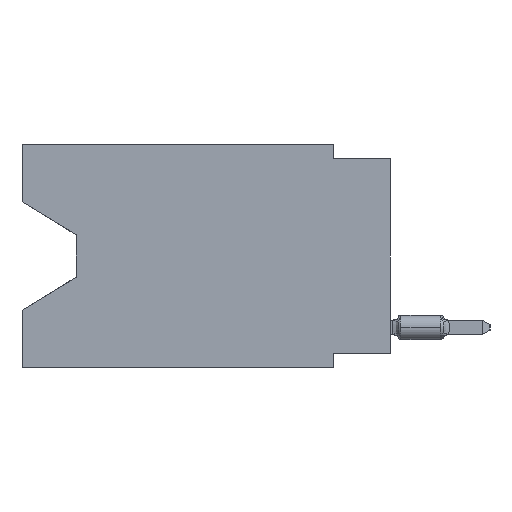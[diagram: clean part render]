
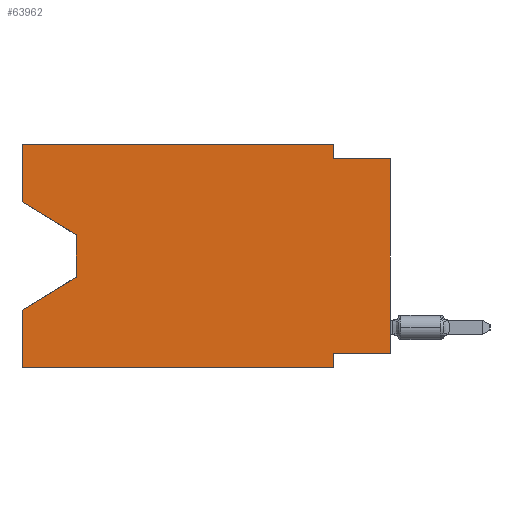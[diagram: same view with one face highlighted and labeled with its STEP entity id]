
A CAD part, left-side view. The second image highlights one B-rep face of the part: STEP entity #63962.
In plain terms, the highlighted planar face has unit normal (-1, 0, 0).
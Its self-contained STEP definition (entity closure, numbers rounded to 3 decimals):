
#1100 = DIRECTION ( 'NONE',  ( 0., -1., 0. ) ) ;
#3446 = VERTEX_POINT ( 'NONE', #51325 ) ;
#4050 = CARTESIAN_POINT ( 'NONE',  ( 0., 16.383, -9.906 ) ) ;
#5705 = DIRECTION ( 'NONE',  ( 0., 1., 0. ) ) ;
#6529 = CARTESIAN_POINT ( 'NONE',  ( 0., 16.383, -2.546 ) ) ;
#7000 = DIRECTION ( 'NONE',  ( 1., 0., 0. ) ) ;
#7169 = CARTESIAN_POINT ( 'NONE',  ( 0., 13.97, -5.893 ) ) ;
#7227 = ORIENTED_EDGE ( 'NONE', *, *, #22013, .T. ) ;
#7622 = DIRECTION ( 'NONE',  ( 0., 0., -1. ) ) ;
#9338 = ORIENTED_EDGE ( 'NONE', *, *, #45527, .F. ) ;
#9466 = ORIENTED_EDGE ( 'NONE', *, *, #44551, .F. ) ;
#9526 = DIRECTION ( 'NONE',  ( 0., -0.855, -0.519 ) ) ;
#13173 = VECTOR ( 'NONE', #13715, 1000. ) ;
#13715 = DIRECTION ( 'NONE',  ( 0., 0., -1. ) ) ;
#14087 = VERTEX_POINT ( 'NONE', #22613 ) ;
#16287 = ORIENTED_EDGE ( 'NONE', *, *, #86094, .F. ) ;
#17542 = LINE ( 'NONE', #64911, #18550 ) ;
#18323 = VERTEX_POINT ( 'NONE', #63926 ) ;
#18550 = VECTOR ( 'NONE', #64053, 1000. ) ;
#19285 = LINE ( 'NONE', #72832, #58833 ) ;
#20139 = CARTESIAN_POINT ( 'NONE',  ( 0., 16.383, 0. ) ) ;
#20149 = VERTEX_POINT ( 'NONE', #28421 ) ;
#20313 = DIRECTION ( 'NONE',  ( 0., -1., 0. ) ) ;
#20867 = CARTESIAN_POINT ( 'NONE',  ( 0., 2.54, 0. ) ) ;
#21386 = LINE ( 'NONE', #41567, #60783 ) ;
#22013 = EDGE_CURVE ( 'NONE', #68593, #73590, #39186, .T. ) ;
#22613 = CARTESIAN_POINT ( 'NONE',  ( 0., 2.54, -9.906 ) ) ;
#23904 = VECTOR ( 'NONE', #28828, 1000. ) ;
#23957 = VECTOR ( 'NONE', #1100, 1000. ) ;
#26957 = ORIENTED_EDGE ( 'NONE', *, *, #59845, .F. ) ;
#27510 = LINE ( 'NONE', #54267, #23904 ) ;
#28421 = CARTESIAN_POINT ( 'NONE',  ( 0., 0., -0.635 ) ) ;
#28681 = VERTEX_POINT ( 'NONE', #39220 ) ;
#28828 = DIRECTION ( 'NONE',  ( 0., 0., -1. ) ) ;
#29266 = ORIENTED_EDGE ( 'NONE', *, *, #60926, .F. ) ;
#30355 = VECTOR ( 'NONE', #7622, 1000. ) ;
#31122 = DIRECTION ( 'NONE',  ( 0., 0., 1. ) ) ;
#33147 = EDGE_CURVE ( 'NONE', #73590, #18323, #21386, .T. ) ;
#33764 = DIRECTION ( 'NONE',  ( 0., 0., -1. ) ) ;
#33945 = CARTESIAN_POINT ( 'NONE',  ( 0., 2.54, -9.906 ) ) ;
#35303 = CARTESIAN_POINT ( 'NONE',  ( 0., 16.383, 0. ) ) ;
#37456 = VERTEX_POINT ( 'NONE', #48938 ) ;
#37685 = CARTESIAN_POINT ( 'NONE',  ( 0., 16.383, 0. ) ) ;
#38250 = CARTESIAN_POINT ( 'NONE',  ( 0., 16.383, 0. ) ) ;
#39143 = ORIENTED_EDGE ( 'NONE', *, *, #33147, .T. ) ;
#39186 = LINE ( 'NONE', #45760, #13173 ) ;
#39220 = CARTESIAN_POINT ( 'NONE',  ( 0., 0., -9.271 ) ) ;
#39267 = EDGE_CURVE ( 'NONE', #47668, #49638, #74366, .T. ) ;
#39638 = CARTESIAN_POINT ( 'NONE',  ( 0., 0., -0.635 ) ) ;
#39765 = EDGE_CURVE ( 'NONE', #83845, #68593, #49464, .T. ) ;
#41567 = CARTESIAN_POINT ( 'NONE',  ( 0., 13.97, -5.893 ) ) ;
#41994 = ORIENTED_EDGE ( 'NONE', *, *, #83602, .F. ) ;
#42689 = EDGE_LOOP ( 'NONE', ( #65002, #7227, #39143, #9338, #83336, #9466, #29266, #73421, #41994, #26957, #80597, #16287 ) ) ;
#44551 = EDGE_CURVE ( 'NONE', #3446, #14087, #73864, .T. ) ;
#45051 = VERTEX_POINT ( 'NONE', #4050 ) ;
#45527 = EDGE_CURVE ( 'NONE', #45051, #18323, #57439, .T. ) ;
#45760 = CARTESIAN_POINT ( 'NONE',  ( 0., 13.97, -4.013 ) ) ;
#47528 = LINE ( 'NONE', #39638, #49148 ) ;
#47668 = VERTEX_POINT ( 'NONE', #76351 ) ;
#47856 = LINE ( 'NONE', #61886, #74213 ) ;
#48711 = DIRECTION ( 'NONE',  ( 0., 0., 1. ) ) ;
#48938 = CARTESIAN_POINT ( 'NONE',  ( 0., 2.54, -0.635 ) ) ;
#49148 = VECTOR ( 'NONE', #20313, 1000. ) ;
#49464 = LINE ( 'NONE', #56043, #79996 ) ;
#49638 = VERTEX_POINT ( 'NONE', #20867 ) ;
#51325 = CARTESIAN_POINT ( 'NONE',  ( 0., 2.54, -9.271 ) ) ;
#52343 = EDGE_CURVE ( 'NONE', #45051, #14087, #17542, .T. ) ;
#53489 = PLANE ( 'NONE',  #70437 ) ;
#54267 = CARTESIAN_POINT ( 'NONE',  ( 0., 2.54, 0. ) ) ;
#56043 = CARTESIAN_POINT ( 'NONE',  ( 0., 16.383, -2.546 ) ) ;
#56861 = CARTESIAN_POINT ( 'NONE',  ( 0., 13.97, -4.013 ) ) ;
#57439 = LINE ( 'NONE', #37685, #78140 ) ;
#57526 = VECTOR ( 'NONE', #65013, 1000. ) ;
#58833 = VECTOR ( 'NONE', #5705, 1000. ) ;
#59845 = EDGE_CURVE ( 'NONE', #49638, #37456, #27510, .T. ) ;
#60783 = VECTOR ( 'NONE', #68330, 1000. ) ;
#60926 = EDGE_CURVE ( 'NONE', #28681, #3446, #19285, .T. ) ;
#61886 = CARTESIAN_POINT ( 'NONE',  ( 0., 0., 0. ) ) ;
#63926 = CARTESIAN_POINT ( 'NONE',  ( 0., 16.383, -7.36 ) ) ;
#63962 = ADVANCED_FACE ( 'NONE', ( #66236 ), #53489, .F. ) ;
#64053 = DIRECTION ( 'NONE',  ( 0., -1., 0. ) ) ;
#64911 = CARTESIAN_POINT ( 'NONE',  ( 0., 16.383, -9.906 ) ) ;
#65002 = ORIENTED_EDGE ( 'NONE', *, *, #39765, .T. ) ;
#65013 = DIRECTION ( 'NONE',  ( 0., 0., 1. ) ) ;
#66236 = FACE_OUTER_BOUND ( 'NONE', #42689, .T. ) ;
#68330 = DIRECTION ( 'NONE',  ( 0., 0.855, -0.519 ) ) ;
#68593 = VERTEX_POINT ( 'NONE', #56861 ) ;
#70437 = AXIS2_PLACEMENT_3D ( 'NONE', #20139, #7000, #33764 ) ;
#72832 = CARTESIAN_POINT ( 'NONE',  ( 0., 0., -9.271 ) ) ;
#73421 = ORIENTED_EDGE ( 'NONE', *, *, #82467, .T. ) ;
#73590 = VERTEX_POINT ( 'NONE', #7169 ) ;
#73864 = LINE ( 'NONE', #33945, #30355 ) ;
#74213 = VECTOR ( 'NONE', #48711, 1000. ) ;
#74366 = LINE ( 'NONE', #35303, #23957 ) ;
#76351 = CARTESIAN_POINT ( 'NONE',  ( 0., 16.383, 0. ) ) ;
#78140 = VECTOR ( 'NONE', #31122, 1000. ) ;
#78620 = LINE ( 'NONE', #38250, #57526 ) ;
#79996 = VECTOR ( 'NONE', #9526, 1000. ) ;
#80597 = ORIENTED_EDGE ( 'NONE', *, *, #39267, .F. ) ;
#82467 = EDGE_CURVE ( 'NONE', #28681, #20149, #47856, .T. ) ;
#83336 = ORIENTED_EDGE ( 'NONE', *, *, #52343, .T. ) ;
#83602 = EDGE_CURVE ( 'NONE', #37456, #20149, #47528, .T. ) ;
#83845 = VERTEX_POINT ( 'NONE', #6529 ) ;
#86094 = EDGE_CURVE ( 'NONE', #83845, #47668, #78620, .T. ) ;
